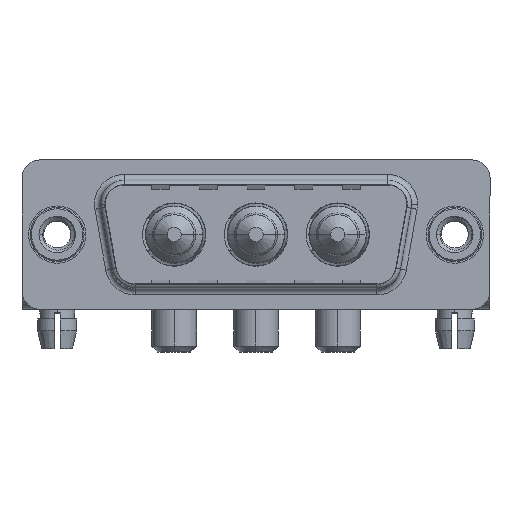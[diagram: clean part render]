
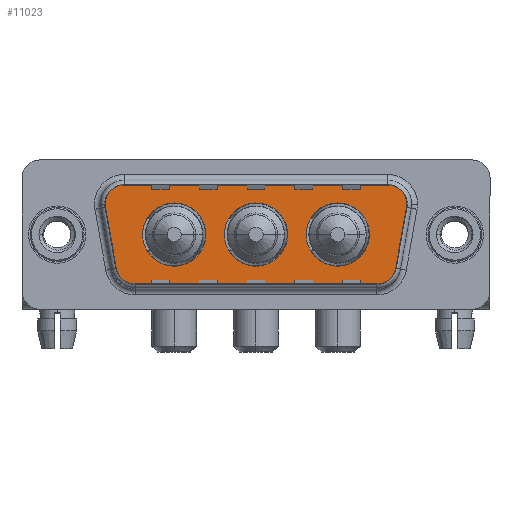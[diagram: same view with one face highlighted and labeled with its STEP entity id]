
A CAD part, top view. The second image highlights one B-rep face of the part: STEP entity #11023.
In plain terms, the highlighted planar face has unit normal (0, 0, 1).
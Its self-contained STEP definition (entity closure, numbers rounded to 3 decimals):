
#127 = EDGE_LOOP ( 'NONE', ( #9372, #6159 ) ) ;
#319 = CARTESIAN_POINT ( 'NONE',  ( 14., 0., 0. ) ) ;
#324 = VECTOR ( 'NONE', #5418, 1000. ) ;
#404 = FACE_BOUND ( 'NONE', #4960, .T. ) ;
#487 = DIRECTION ( 'NONE',  ( 0., 0., 1. ) ) ;
#545 = ORIENTED_EDGE ( 'NONE', *, *, #1154, .T. ) ;
#791 = VERTEX_POINT ( 'NONE', #12204 ) ;
#930 = ORIENTED_EDGE ( 'NONE', *, *, #15851, .F. ) ;
#982 = DIRECTION ( 'NONE',  ( 1., 0., 0. ) ) ;
#1031 = ORIENTED_EDGE ( 'NONE', *, *, #15555, .F. ) ;
#1154 = EDGE_CURVE ( 'NONE', #2568, #12327, #15370, .T. ) ;
#1227 = DIRECTION ( 'NONE',  ( 0., 0., 1. ) ) ;
#1237 = EDGE_CURVE ( 'NONE', #8776, #16050, #14037, .T. ) ;
#1358 = DIRECTION ( 'NONE',  ( -1., 0., 0. ) ) ;
#1384 = ORIENTED_EDGE ( 'NONE', *, *, #3255, .T. ) ;
#1756 = EDGE_CURVE ( 'NONE', #791, #9355, #15872, .T. ) ;
#1811 = DIRECTION ( 'NONE',  ( 1., 0., 0. ) ) ;
#2204 = DIRECTION ( 'NONE',  ( 0., 0., 1. ) ) ;
#2263 = VERTEX_POINT ( 'NONE', #13983 ) ;
#2470 = EDGE_CURVE ( 'NONE', #11616, #14667, #5178, .T. ) ;
#2568 = VERTEX_POINT ( 'NONE', #16007 ) ;
#2851 = LINE ( 'NONE', #15398, #12151 ) ;
#3025 = CARTESIAN_POINT ( 'NONE',  ( 23.5, 0., 0. ) ) ;
#3162 = AXIS2_PLACEMENT_3D ( 'NONE', #3610, #11933, #8025 ) ;
#3255 = EDGE_CURVE ( 'NONE', #9417, #8776, #5036, .T. ) ;
#3289 = DIRECTION ( 'NONE',  ( 1., 0., 0. ) ) ;
#3610 = CARTESIAN_POINT ( 'NONE',  ( 9.8, 0., 0. ) ) ;
#3648 = AXIS2_PLACEMENT_3D ( 'NONE', #12364, #15810, #982 ) ;
#3963 = AXIS2_PLACEMENT_3D ( 'NONE', #9525, #13272, #1811 ) ;
#4147 = DIRECTION ( 'NONE',  ( 0., 0., 1. ) ) ;
#4577 = EDGE_LOOP ( 'NONE', ( #9295, #1031 ) ) ;
#4651 = CARTESIAN_POINT ( 'NONE',  ( 29.889, 2.9, 0. ) ) ;
#4844 = CARTESIAN_POINT ( 'NONE',  ( 5.411, 4.9, 0. ) ) ;
#4941 = CARTESIAN_POINT ( 'NONE',  ( 5.411, 2.9, 0. ) ) ;
#4960 = EDGE_LOOP ( 'NONE', ( #10344, #930 ) ) ;
#5019 = CARTESIAN_POINT ( 'NONE',  ( 27.889, 2.9, 0. ) ) ;
#5036 = CIRCLE ( 'NONE', #11137, 2. ) ;
#5178 = LINE ( 'NONE', #9074, #8200 ) ;
#5316 = ORIENTED_EDGE ( 'NONE', *, *, #9178, .T. ) ;
#5418 = DIRECTION ( 'NONE',  ( 1., 0., 0. ) ) ;
#5552 = DIRECTION ( 'NONE',  ( 1., 0., 0. ) ) ;
#5650 = ORIENTED_EDGE ( 'NONE', *, *, #8560, .T. ) ;
#5696 = DIRECTION ( 'NONE',  ( 0., 0., 1. ) ) ;
#5707 = CARTESIAN_POINT ( 'NONE',  ( 27.889, 2.9, 0. ) ) ;
#6159 = ORIENTED_EDGE ( 'NONE', *, *, #13505, .F. ) ;
#6276 = DIRECTION ( 'NONE',  ( 0., 0., 1. ) ) ;
#6776 = PLANE ( 'NONE',  #9689 ) ;
#6985 = ORIENTED_EDGE ( 'NONE', *, *, #1237, .T. ) ;
#7054 = CARTESIAN_POINT ( 'NONE',  ( 6.434, -4.9, 0. ) ) ;
#7111 = VERTEX_POINT ( 'NONE', #11709 ) ;
#7250 = ORIENTED_EDGE ( 'NONE', *, *, #8152, .T. ) ;
#7326 = CIRCLE ( 'NONE', #11073, 2. ) ;
#7331 = DIRECTION ( 'NONE',  ( 1., 0., 0. ) ) ;
#7376 = VECTOR ( 'NONE', #11677, 1000. ) ;
#7602 = CARTESIAN_POINT ( 'NONE',  ( 29.859, 2.553, 0. ) ) ;
#7665 = AXIS2_PLACEMENT_3D ( 'NONE', #5707, #10775, #15843 ) ;
#7699 = DIRECTION ( 'NONE',  ( 1., 0., 0. ) ) ;
#7952 = FACE_BOUND ( 'NONE', #4577, .T. ) ;
#8025 = DIRECTION ( 'NONE',  ( 1., 0., 0. ) ) ;
#8054 = CARTESIAN_POINT ( 'NONE',  ( 20.85, 0., 0. ) ) ;
#8076 = DIRECTION ( 'NONE',  ( 0., 0., 1. ) ) ;
#8152 = EDGE_CURVE ( 'NONE', #7111, #2568, #8154, .T. ) ;
#8154 = LINE ( 'NONE', #7054, #324 ) ;
#8189 = AXIS2_PLACEMENT_3D ( 'NONE', #12612, #1227, #11369 ) ;
#8200 = VECTOR ( 'NONE', #15390, 1000. ) ;
#8264 = CARTESIAN_POINT ( 'NONE',  ( 3.441, 2.553, 0. ) ) ;
#8371 = CARTESIAN_POINT ( 'NONE',  ( 7.15, 0., 0. ) ) ;
#8560 = EDGE_CURVE ( 'NONE', #10340, #11616, #7326, .T. ) ;
#8776 = VERTEX_POINT ( 'NONE', #4651 ) ;
#9074 = CARTESIAN_POINT ( 'NONE',  ( 3.441, 2.553, 0. ) ) ;
#9178 = EDGE_CURVE ( 'NONE', #14667, #7111, #10909, .T. ) ;
#9196 = FACE_BOUND ( 'NONE', #127, .T. ) ;
#9231 = CARTESIAN_POINT ( 'NONE',  ( 28.836, -3.247, 0. ) ) ;
#9295 = ORIENTED_EDGE ( 'NONE', *, *, #12044, .F. ) ;
#9355 = VERTEX_POINT ( 'NONE', #8371 ) ;
#9372 = ORIENTED_EDGE ( 'NONE', *, *, #14383, .F. ) ;
#9417 = VERTEX_POINT ( 'NONE', #7602 ) ;
#9525 = CARTESIAN_POINT ( 'NONE',  ( 26.866, -2.9, 0. ) ) ;
#9587 = VERTEX_POINT ( 'NONE', #319 ) ;
#9689 = AXIS2_PLACEMENT_3D ( 'NONE', #11298, #487, #5552 ) ;
#9910 = CARTESIAN_POINT ( 'NONE',  ( 27.889, 4.9, 0. ) ) ;
#10340 = VERTEX_POINT ( 'NONE', #4844 ) ;
#10344 = ORIENTED_EDGE ( 'NONE', *, *, #1756, .F. ) ;
#10775 = DIRECTION ( 'NONE',  ( 0., 0., 1. ) ) ;
#10909 = CIRCLE ( 'NONE', #15145, 2. ) ;
#10956 = VERTEX_POINT ( 'NONE', #11772 ) ;
#11023 = ADVANCED_FACE ( 'NONE', ( #9196, #7952, #404, #14356 ), #6776, .T. ) ;
#11044 = CIRCLE ( 'NONE', #14499, 2.65 ) ;
#11073 = AXIS2_PLACEMENT_3D ( 'NONE', #4941, #2204, #7331 ) ;
#11137 = AXIS2_PLACEMENT_3D ( 'NONE', #5019, #12492, #11242 ) ;
#11242 = DIRECTION ( 'NONE',  ( -1., 0., 0. ) ) ;
#11298 = CARTESIAN_POINT ( 'NONE',  ( 26.866, -2.9, 0. ) ) ;
#11369 = DIRECTION ( 'NONE',  ( 1., 0., 0. ) ) ;
#11492 = CARTESIAN_POINT ( 'NONE',  ( 4.464, -3.247, 0. ) ) ;
#11616 = VERTEX_POINT ( 'NONE', #8264 ) ;
#11617 = AXIS2_PLACEMENT_3D ( 'NONE', #12443, #6276, #7699 ) ;
#11639 = AXIS2_PLACEMENT_3D ( 'NONE', #13172, #5696, #3289 ) ;
#11666 = ORIENTED_EDGE ( 'NONE', *, *, #14316, .T. ) ;
#11677 = DIRECTION ( 'NONE',  ( 0.174, 0.985, 0. ) ) ;
#11709 = CARTESIAN_POINT ( 'NONE',  ( 6.434, -4.9, 0. ) ) ;
#11772 = CARTESIAN_POINT ( 'NONE',  ( 26.15, 0., 0. ) ) ;
#11873 = ORIENTED_EDGE ( 'NONE', *, *, #14675, .T. ) ;
#11933 = DIRECTION ( 'NONE',  ( 0., 0., 1. ) ) ;
#12044 = EDGE_CURVE ( 'NONE', #10956, #12948, #11044, .T. ) ;
#12151 = VECTOR ( 'NONE', #1358, 1000. ) ;
#12204 = CARTESIAN_POINT ( 'NONE',  ( 12.45, 0., 0. ) ) ;
#12327 = VERTEX_POINT ( 'NONE', #9231 ) ;
#12364 = CARTESIAN_POINT ( 'NONE',  ( 16.65, 0., 0. ) ) ;
#12410 = EDGE_LOOP ( 'NONE', ( #545, #11666, #1384, #6985, #11873, #5650, #14323, #5316, #7250 ) ) ;
#12443 = CARTESIAN_POINT ( 'NONE',  ( 9.8, 0., 0. ) ) ;
#12492 = DIRECTION ( 'NONE',  ( 0., 0., 1. ) ) ;
#12612 = CARTESIAN_POINT ( 'NONE',  ( 23.5, 0., 0. ) ) ;
#12935 = CIRCLE ( 'NONE', #3648, 2.65 ) ;
#12948 = VERTEX_POINT ( 'NONE', #8054 ) ;
#13172 = CARTESIAN_POINT ( 'NONE',  ( 16.65, 0., 0. ) ) ;
#13272 = DIRECTION ( 'NONE',  ( 0., 0., 1. ) ) ;
#13482 = CIRCLE ( 'NONE', #11639, 2.65 ) ;
#13505 = EDGE_CURVE ( 'NONE', #9587, #2263, #12935, .T. ) ;
#13754 = CIRCLE ( 'NONE', #3162, 2.65 ) ;
#13983 = CARTESIAN_POINT ( 'NONE',  ( 19.3, 0., 0. ) ) ;
#14037 = CIRCLE ( 'NONE', #7665, 2. ) ;
#14157 = CARTESIAN_POINT ( 'NONE',  ( 29.859, 2.553, 0. ) ) ;
#14187 = DIRECTION ( 'NONE',  ( -1., 0., 0. ) ) ;
#14293 = CIRCLE ( 'NONE', #8189, 2.65 ) ;
#14316 = EDGE_CURVE ( 'NONE', #12327, #9417, #15673, .T. ) ;
#14323 = ORIENTED_EDGE ( 'NONE', *, *, #2470, .T. ) ;
#14356 = FACE_OUTER_BOUND ( 'NONE', #12410, .T. ) ;
#14383 = EDGE_CURVE ( 'NONE', #2263, #9587, #13482, .T. ) ;
#14499 = AXIS2_PLACEMENT_3D ( 'NONE', #3025, #8076, #14556 ) ;
#14556 = DIRECTION ( 'NONE',  ( 1., 0., 0. ) ) ;
#14667 = VERTEX_POINT ( 'NONE', #11492 ) ;
#14675 = EDGE_CURVE ( 'NONE', #16050, #10340, #2851, .T. ) ;
#15145 = AXIS2_PLACEMENT_3D ( 'NONE', #15443, #4147, #14187 ) ;
#15370 = CIRCLE ( 'NONE', #3963, 2. ) ;
#15390 = DIRECTION ( 'NONE',  ( 0.174, -0.985, 0. ) ) ;
#15398 = CARTESIAN_POINT ( 'NONE',  ( 5.411, 4.9, 0. ) ) ;
#15443 = CARTESIAN_POINT ( 'NONE',  ( 6.434, -2.9, 0. ) ) ;
#15555 = EDGE_CURVE ( 'NONE', #12948, #10956, #14293, .T. ) ;
#15673 = LINE ( 'NONE', #14157, #7376 ) ;
#15810 = DIRECTION ( 'NONE',  ( 0., 0., 1. ) ) ;
#15843 = DIRECTION ( 'NONE',  ( -1., 0., 0. ) ) ;
#15851 = EDGE_CURVE ( 'NONE', #9355, #791, #13754, .T. ) ;
#15872 = CIRCLE ( 'NONE', #11617, 2.65 ) ;
#16007 = CARTESIAN_POINT ( 'NONE',  ( 26.866, -4.9, 0. ) ) ;
#16050 = VERTEX_POINT ( 'NONE', #9910 ) ;
